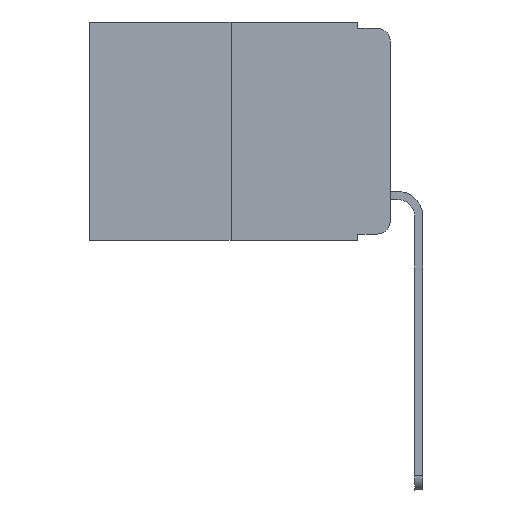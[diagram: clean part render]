
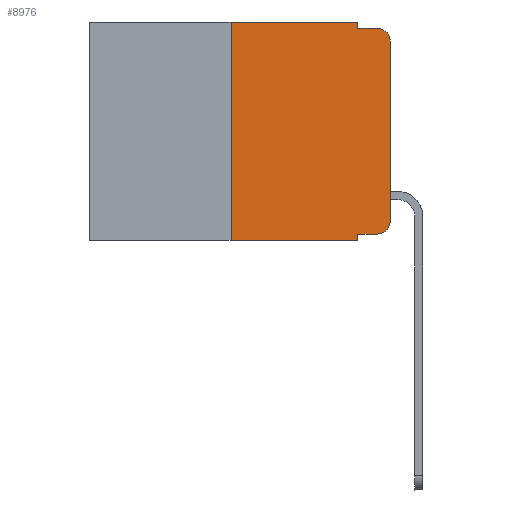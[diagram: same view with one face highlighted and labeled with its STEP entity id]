
A CAD part, left-side view. The second image highlights one B-rep face of the part: STEP entity #8976.
In plain terms, the highlighted planar face has unit normal (-1, 0, 0).
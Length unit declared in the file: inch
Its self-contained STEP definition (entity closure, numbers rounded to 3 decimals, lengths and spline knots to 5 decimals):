
#133 = VERTEX_POINT ( 'NONE', #9073 ) ;
#169 = DIRECTION ( 'NONE',  ( 0., 0., -1. ) ) ;
#299 = VERTEX_POINT ( 'NONE', #5700 ) ;
#332 = CIRCLE ( 'NONE', #1891, 0.02 ) ;
#375 = ORIENTED_EDGE ( 'NONE', *, *, #2417, .T. ) ;
#425 = DIRECTION ( 'NONE',  ( 0., 0., 1. ) ) ;
#835 = DIRECTION ( 'NONE',  ( 0., 0., -1. ) ) ;
#879 = LINE ( 'NONE', #8483, #5705 ) ;
#1155 = CIRCLE ( 'NONE', #2270, 0.02 ) ;
#1330 = EDGE_CURVE ( 'NONE', #5460, #7616, #8036, .T. ) ;
#1377 = VERTEX_POINT ( 'NONE', #13732 ) ;
#1485 = CARTESIAN_POINT ( 'NONE',  ( 0., 0., 0. ) ) ;
#1736 = CARTESIAN_POINT ( 'NONE',  ( 0., 0.02, -0.313 ) ) ;
#1748 = DIRECTION ( 'NONE',  ( 0., -1., 0. ) ) ;
#1799 = CARTESIAN_POINT ( 'NONE',  ( 0., 0.02, -0.03 ) ) ;
#1801 = VERTEX_POINT ( 'NONE', #4880 ) ;
#1891 = AXIS2_PLACEMENT_3D ( 'NONE', #1799, #9198, #835 ) ;
#1927 = VECTOR ( 'NONE', #5330, 39.37008 ) ;
#2270 = AXIS2_PLACEMENT_3D ( 'NONE', #1736, #13511, #10518 ) ;
#2415 = EDGE_CURVE ( 'NONE', #1801, #4987, #9395, .T. ) ;
#2417 = EDGE_CURVE ( 'NONE', #1377, #10602, #332, .T. ) ;
#2924 = ORIENTED_EDGE ( 'NONE', *, *, #2415, .F. ) ;
#3673 = VECTOR ( 'NONE', #9263, 39.37008 ) ;
#3741 = VECTOR ( 'NONE', #1748, 39.37008 ) ;
#3942 = CARTESIAN_POINT ( 'NONE',  ( 0., 0.051, 0. ) ) ;
#4247 = CARTESIAN_POINT ( 'NONE',  ( 0., 0.473, -0.343 ) ) ;
#4365 = PLANE ( 'NONE',  #8102 ) ;
#4448 = EDGE_CURVE ( 'NONE', #299, #6487, #1155, .T. ) ;
#4675 = CARTESIAN_POINT ( 'NONE',  ( 0., 0.02, -0.01 ) ) ;
#4689 = ORIENTED_EDGE ( 'NONE', *, *, #1330, .F. ) ;
#4702 = ORIENTED_EDGE ( 'NONE', *, *, #9717, .T. ) ;
#4880 = CARTESIAN_POINT ( 'NONE',  ( 0., 0.051, -0.333 ) ) ;
#4932 = CARTESIAN_POINT ( 'NONE',  ( 0., 0.051, -0.01 ) ) ;
#4956 = CARTESIAN_POINT ( 'NONE',  ( 0., 0.051, 0. ) ) ;
#4987 = VERTEX_POINT ( 'NONE', #5401 ) ;
#5063 = DIRECTION ( 'NONE',  ( 0., -1., 0. ) ) ;
#5330 = DIRECTION ( 'NONE',  ( 0., 0., 1. ) ) ;
#5358 = VERTEX_POINT ( 'NONE', #12481 ) ;
#5401 = CARTESIAN_POINT ( 'NONE',  ( 0., 0.051, -0.343 ) ) ;
#5460 = VERTEX_POINT ( 'NONE', #6500 ) ;
#5700 = CARTESIAN_POINT ( 'NONE',  ( 0., 0.02, -0.333 ) ) ;
#5705 = VECTOR ( 'NONE', #5063, 39.37008 ) ;
#6294 = VECTOR ( 'NONE', #9816, 39.37008 ) ;
#6487 = VERTEX_POINT ( 'NONE', #12796 ) ;
#6500 = CARTESIAN_POINT ( 'NONE',  ( 0., 0.25, 0. ) ) ;
#7616 = VERTEX_POINT ( 'NONE', #3942 ) ;
#7947 = DIRECTION ( 'NONE',  ( 0., -1., 0. ) ) ;
#8036 = LINE ( 'NONE', #10193, #3741 ) ;
#8099 = EDGE_CURVE ( 'NONE', #7616, #133, #12898, .T. ) ;
#8102 = AXIS2_PLACEMENT_3D ( 'NONE', #9513, #9576, #169 ) ;
#8483 = CARTESIAN_POINT ( 'NONE',  ( 0., 0.051, -0.333 ) ) ;
#8976 = ADVANCED_FACE ( 'NONE', ( #9647 ), #4365, .F. ) ;
#9073 = CARTESIAN_POINT ( 'NONE',  ( 0., 0.051, -0.01 ) ) ;
#9198 = DIRECTION ( 'NONE',  ( -1., 0., 0. ) ) ;
#9263 = DIRECTION ( 'NONE',  ( 0., 0., -1. ) ) ;
#9395 = LINE ( 'NONE', #4956, #3673 ) ;
#9417 = EDGE_LOOP ( 'NONE', ( #10708, #375, #11961, #10103, #4689, #12537, #4702, #2924, #9992, #12520 ) ) ;
#9490 = EDGE_CURVE ( 'NONE', #6487, #1377, #10885, .T. ) ;
#9513 = CARTESIAN_POINT ( 'NONE',  ( 0., 0.473, 0. ) ) ;
#9576 = DIRECTION ( 'NONE',  ( 1., 0., 0. ) ) ;
#9647 = FACE_OUTER_BOUND ( 'NONE', #9417, .T. ) ;
#9717 = EDGE_CURVE ( 'NONE', #5358, #4987, #13789, .T. ) ;
#9816 = DIRECTION ( 'NONE',  ( 0., 0., -1. ) ) ;
#9885 = VECTOR ( 'NONE', #10655, 39.37008 ) ;
#9992 = ORIENTED_EDGE ( 'NONE', *, *, #12533, .T. ) ;
#10103 = ORIENTED_EDGE ( 'NONE', *, *, #8099, .F. ) ;
#10193 = CARTESIAN_POINT ( 'NONE',  ( 0., 0.473, 0. ) ) ;
#10518 = DIRECTION ( 'NONE',  ( 0., 0., -1. ) ) ;
#10602 = VERTEX_POINT ( 'NONE', #4675 ) ;
#10624 = CARTESIAN_POINT ( 'NONE',  ( 0., 0.25, 0. ) ) ;
#10655 = DIRECTION ( 'NONE',  ( 0., -1., 0. ) ) ;
#10708 = ORIENTED_EDGE ( 'NONE', *, *, #9490, .T. ) ;
#10885 = LINE ( 'NONE', #1485, #11670 ) ;
#10891 = LINE ( 'NONE', #10624, #1927 ) ;
#11670 = VECTOR ( 'NONE', #425, 39.37008 ) ;
#11961 = ORIENTED_EDGE ( 'NONE', *, *, #13599, .F. ) ;
#12481 = CARTESIAN_POINT ( 'NONE',  ( 0., 0.25, -0.343 ) ) ;
#12520 = ORIENTED_EDGE ( 'NONE', *, *, #4448, .T. ) ;
#12533 = EDGE_CURVE ( 'NONE', #1801, #299, #879, .T. ) ;
#12537 = ORIENTED_EDGE ( 'NONE', *, *, #13095, .F. ) ;
#12796 = CARTESIAN_POINT ( 'NONE',  ( 0., 0., -0.313 ) ) ;
#12824 = CARTESIAN_POINT ( 'NONE',  ( 0., 0.051, 0. ) ) ;
#12898 = LINE ( 'NONE', #12824, #6294 ) ;
#13095 = EDGE_CURVE ( 'NONE', #5358, #5460, #10891, .T. ) ;
#13300 = LINE ( 'NONE', #4932, #13512 ) ;
#13511 = DIRECTION ( 'NONE',  ( -1., 0., 0. ) ) ;
#13512 = VECTOR ( 'NONE', #7947, 39.37008 ) ;
#13599 = EDGE_CURVE ( 'NONE', #133, #10602, #13300, .T. ) ;
#13732 = CARTESIAN_POINT ( 'NONE',  ( 0., 0., -0.03 ) ) ;
#13789 = LINE ( 'NONE', #4247, #9885 ) ;
